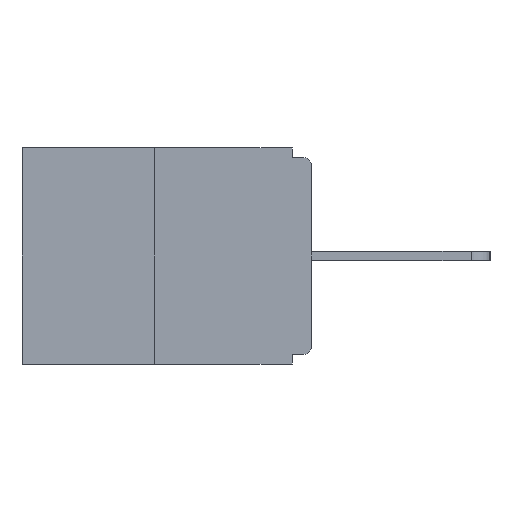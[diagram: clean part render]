
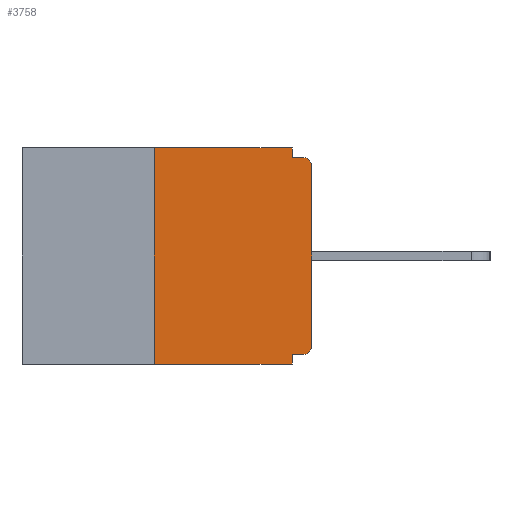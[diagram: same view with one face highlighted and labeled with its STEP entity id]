
A CAD part, left-side view. The second image highlights one B-rep face of the part: STEP entity #3758.
In plain terms, the highlighted planar face has unit normal (-1, 0, 0).
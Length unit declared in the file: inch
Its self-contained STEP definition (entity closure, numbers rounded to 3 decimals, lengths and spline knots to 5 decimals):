
#79 = DIRECTION ( 'NONE',  ( 0., 0., -1. ) ) ;
#93 = VECTOR ( 'NONE', #7667, 39.37008 ) ;
#231 = CARTESIAN_POINT ( 'NONE',  ( 0., 0.031, 0. ) ) ;
#394 = VERTEX_POINT ( 'NONE', #3568 ) ;
#760 = VECTOR ( 'NONE', #13056, 39.37008 ) ;
#929 = ORIENTED_EDGE ( 'NONE', *, *, #2541, .F. ) ;
#1273 = EDGE_CURVE ( 'NONE', #10761, #7390, #9142, .T. ) ;
#1298 = EDGE_CURVE ( 'NONE', #14530, #394, #8559, .T. ) ;
#1301 = VERTEX_POINT ( 'NONE', #5171 ) ;
#1330 = ORIENTED_EDGE ( 'NONE', *, *, #2516, .F. ) ;
#1346 = CARTESIAN_POINT ( 'NONE',  ( 0., 0.46, 0. ) ) ;
#1710 = DIRECTION ( 'NONE',  ( 0., -1., 0. ) ) ;
#2203 = CARTESIAN_POINT ( 'NONE',  ( 0., 0.25, 0. ) ) ;
#2291 = EDGE_LOOP ( 'NONE', ( #3854, #19791, #17521, #1330, #929, #16418, #5132, #14326, #6847, #15014 ) ) ;
#2516 = EDGE_CURVE ( 'NONE', #16590, #15672, #10647, .T. ) ;
#2541 = EDGE_CURVE ( 'NONE', #15620, #16590, #20527, .T. ) ;
#3314 = DIRECTION ( 'NONE',  ( -1., 0., 0. ) ) ;
#3568 = CARTESIAN_POINT ( 'NONE',  ( 0., 0., -0.03 ) ) ;
#3578 = VECTOR ( 'NONE', #10980, 39.37008 ) ;
#3758 = ADVANCED_FACE ( 'NONE', ( #4731 ), #6676, .F. ) ;
#3854 = ORIENTED_EDGE ( 'NONE', *, *, #6690, .F. ) ;
#4515 = DIRECTION ( 'NONE',  ( 0., -1., 0. ) ) ;
#4731 = FACE_OUTER_BOUND ( 'NONE', #2291, .T. ) ;
#4803 = EDGE_CURVE ( 'NONE', #1301, #10761, #6593, .T. ) ;
#4846 = VECTOR ( 'NONE', #4515, 39.37008 ) ;
#5060 = CARTESIAN_POINT ( 'NONE',  ( 0., 0.015, -0.313 ) ) ;
#5110 = LINE ( 'NONE', #16612, #4846 ) ;
#5132 = ORIENTED_EDGE ( 'NONE', *, *, #1298, .T. ) ;
#5171 = CARTESIAN_POINT ( 'NONE',  ( 0., 0.031, 0. ) ) ;
#5355 = CARTESIAN_POINT ( 'NONE',  ( 0., 0.46, 0. ) ) ;
#6593 = LINE ( 'NONE', #231, #3578 ) ;
#6676 = PLANE ( 'NONE',  #9420 ) ;
#6690 = EDGE_CURVE ( 'NONE', #17856, #1301, #10832, .T. ) ;
#6767 = CARTESIAN_POINT ( 'NONE',  ( 0., 0.25, -0.343 ) ) ;
#6847 = ORIENTED_EDGE ( 'NONE', *, *, #1273, .F. ) ;
#7390 = VERTEX_POINT ( 'NONE', #8163 ) ;
#7667 = DIRECTION ( 'NONE',  ( 0., 0., -1. ) ) ;
#8163 = CARTESIAN_POINT ( 'NONE',  ( 0., 0.015, -0.015 ) ) ;
#8277 = CARTESIAN_POINT ( 'NONE',  ( 0., 0.031, -0.343 ) ) ;
#8559 = LINE ( 'NONE', #11536, #12757 ) ;
#9142 = LINE ( 'NONE', #22078, #14136 ) ;
#9420 = AXIS2_PLACEMENT_3D ( 'NONE', #1346, #18976, #18899 ) ;
#9575 = CARTESIAN_POINT ( 'NONE',  ( 0., 0.031, -0.015 ) ) ;
#10159 = EDGE_CURVE ( 'NONE', #15620, #14530, #11354, .T. ) ;
#10647 = LINE ( 'NONE', #13260, #93 ) ;
#10761 = VERTEX_POINT ( 'NONE', #9575 ) ;
#10832 = LINE ( 'NONE', #5355, #14149 ) ;
#10980 = DIRECTION ( 'NONE',  ( 0., 0., -1. ) ) ;
#11354 = CIRCLE ( 'NONE', #13168, 0.015 ) ;
#11536 = CARTESIAN_POINT ( 'NONE',  ( 0., 0., 0. ) ) ;
#11641 = CARTESIAN_POINT ( 'NONE',  ( 0., 0.015, -0.328 ) ) ;
#12524 = AXIS2_PLACEMENT_3D ( 'NONE', #13935, #3314, #79 ) ;
#12757 = VECTOR ( 'NONE', #15082, 39.37008 ) ;
#13056 = DIRECTION ( 'NONE',  ( 0., 0., 1. ) ) ;
#13168 = AXIS2_PLACEMENT_3D ( 'NONE', #5060, #22645, #15605 ) ;
#13260 = CARTESIAN_POINT ( 'NONE',  ( 0., 0.031, -0.343 ) ) ;
#13935 = CARTESIAN_POINT ( 'NONE',  ( 0., 0.015, -0.03 ) ) ;
#14136 = VECTOR ( 'NONE', #22302, 39.37008 ) ;
#14149 = VECTOR ( 'NONE', #1710, 39.37008 ) ;
#14249 = EDGE_CURVE ( 'NONE', #20894, #17856, #18171, .T. ) ;
#14326 = ORIENTED_EDGE ( 'NONE', *, *, #19976, .T. ) ;
#14530 = VERTEX_POINT ( 'NONE', #21562 ) ;
#14822 = CARTESIAN_POINT ( 'NONE',  ( 0., 0.031, -0.328 ) ) ;
#15014 = ORIENTED_EDGE ( 'NONE', *, *, #4803, .F. ) ;
#15082 = DIRECTION ( 'NONE',  ( 0., 0., 1. ) ) ;
#15605 = DIRECTION ( 'NONE',  ( 0., 0., -1. ) ) ;
#15620 = VERTEX_POINT ( 'NONE', #11641 ) ;
#15672 = VERTEX_POINT ( 'NONE', #8277 ) ;
#16418 = ORIENTED_EDGE ( 'NONE', *, *, #10159, .T. ) ;
#16590 = VERTEX_POINT ( 'NONE', #14822 ) ;
#16612 = CARTESIAN_POINT ( 'NONE',  ( 0., 0.46, -0.343 ) ) ;
#16692 = VECTOR ( 'NONE', #20233, 39.37008 ) ;
#16801 = CARTESIAN_POINT ( 'NONE',  ( 0., 0., -0.328 ) ) ;
#17521 = ORIENTED_EDGE ( 'NONE', *, *, #18420, .T. ) ;
#17856 = VERTEX_POINT ( 'NONE', #22476 ) ;
#18171 = LINE ( 'NONE', #2203, #760 ) ;
#18420 = EDGE_CURVE ( 'NONE', #20894, #15672, #5110, .T. ) ;
#18899 = DIRECTION ( 'NONE',  ( 0., 0., -1. ) ) ;
#18976 = DIRECTION ( 'NONE',  ( 1., 0., 0. ) ) ;
#19791 = ORIENTED_EDGE ( 'NONE', *, *, #14249, .F. ) ;
#19976 = EDGE_CURVE ( 'NONE', #394, #7390, #20493, .T. ) ;
#20233 = DIRECTION ( 'NONE',  ( 0., 1., 0. ) ) ;
#20493 = CIRCLE ( 'NONE', #12524, 0.015 ) ;
#20527 = LINE ( 'NONE', #16801, #16692 ) ;
#20894 = VERTEX_POINT ( 'NONE', #6767 ) ;
#21562 = CARTESIAN_POINT ( 'NONE',  ( 0., 0., -0.313 ) ) ;
#22078 = CARTESIAN_POINT ( 'NONE',  ( 0., 0., -0.015 ) ) ;
#22302 = DIRECTION ( 'NONE',  ( 0., -1., 0. ) ) ;
#22476 = CARTESIAN_POINT ( 'NONE',  ( 0., 0.25, 0. ) ) ;
#22645 = DIRECTION ( 'NONE',  ( -1., 0., 0. ) ) ;
